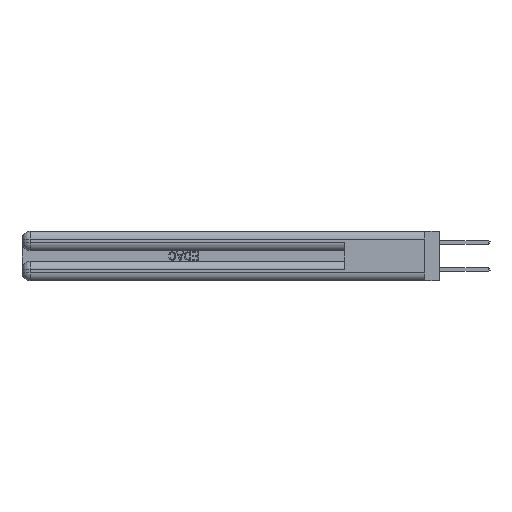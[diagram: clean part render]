
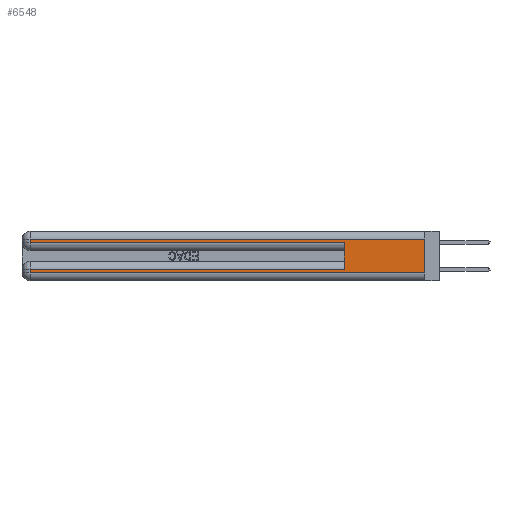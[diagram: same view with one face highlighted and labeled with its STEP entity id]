
A CAD part, left-side view. The second image highlights one B-rep face of the part: STEP entity #6548.
In plain terms, the highlighted planar face has unit normal (-1, 0, 0).
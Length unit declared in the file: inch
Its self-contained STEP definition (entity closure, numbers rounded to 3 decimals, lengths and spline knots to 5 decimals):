
#258 = LINE ( 'NONE', #27085, #29530 ) ;
#1089 = VERTEX_POINT ( 'NONE', #24024 ) ;
#1900 = VERTEX_POINT ( 'NONE', #43409 ) ;
#3963 = VECTOR ( 'NONE', #14091, 39.37008 ) ;
#4613 = CARTESIAN_POINT ( 'NONE',  ( 0., 0., 0.285 ) ) ;
#5064 = DIRECTION ( 'NONE',  ( 0., -1., 0. ) ) ;
#5409 = VERTEX_POINT ( 'NONE', #17122 ) ;
#6548 = ADVANCED_FACE ( 'NONE', ( #34229 ), #28766, .F. ) ;
#7283 = ORIENTED_EDGE ( 'NONE', *, *, #45114, .T. ) ;
#7579 = EDGE_CURVE ( 'NONE', #17850, #36302, #11174, .T. ) ;
#8300 = DIRECTION ( 'NONE',  ( 0., -1., 0. ) ) ;
#8536 = EDGE_LOOP ( 'NONE', ( #27753, #34011, #43330, #7283, #33862, #44814, #28402, #41227 ) ) ;
#9392 = DIRECTION ( 'NONE',  ( 0., 1., 0. ) ) ;
#9418 = EDGE_CURVE ( 'NONE', #31001, #5409, #35344, .T. ) ;
#10345 = CARTESIAN_POINT ( 'NONE',  ( 0., 0., 0.31 ) ) ;
#10462 = DIRECTION ( 'NONE',  ( 0., 0., -1. ) ) ;
#11174 = LINE ( 'NONE', #46698, #30667 ) ;
#11212 = EDGE_CURVE ( 'NONE', #1900, #1089, #258, .T. ) ;
#12594 = CARTESIAN_POINT ( 'NONE',  ( 0., 0.6, 0.145 ) ) ;
#12861 = VECTOR ( 'NONE', #8300, 39.37008 ) ;
#13589 = VERTEX_POINT ( 'NONE', #28543 ) ;
#14091 = DIRECTION ( 'NONE',  ( 0., 1., 0. ) ) ;
#15012 = CARTESIAN_POINT ( 'NONE',  ( 0., 2.94, 0.285 ) ) ;
#15238 = VERTEX_POINT ( 'NONE', #45117 ) ;
#15394 = LINE ( 'NONE', #41301, #33690 ) ;
#17037 = EDGE_CURVE ( 'NONE', #15238, #1089, #15394, .T. ) ;
#17122 = CARTESIAN_POINT ( 'NONE',  ( 0., 2.94, 0.085 ) ) ;
#17517 = DIRECTION ( 'NONE',  ( 0., 0., -1. ) ) ;
#17767 = CARTESIAN_POINT ( 'NONE',  ( 0., 0., 0.37 ) ) ;
#17850 = VERTEX_POINT ( 'NONE', #24314 ) ;
#20043 = DIRECTION ( 'NONE',  ( 0., 0., 1. ) ) ;
#20047 = EDGE_CURVE ( 'NONE', #5409, #1900, #39199, .T. ) ;
#20889 = DIRECTION ( 'NONE',  ( 0., 0., -1. ) ) ;
#22675 = LINE ( 'NONE', #4613, #12861 ) ;
#24024 = CARTESIAN_POINT ( 'NONE',  ( 0., 0., 0.06 ) ) ;
#24314 = CARTESIAN_POINT ( 'NONE',  ( 0., 2.94, 0.31 ) ) ;
#25640 = VECTOR ( 'NONE', #9392, 39.37008 ) ;
#26777 = DIRECTION ( 'NONE',  ( 0., 0., -1. ) ) ;
#27085 = CARTESIAN_POINT ( 'NONE',  ( 0., 0., 0.06 ) ) ;
#27753 = ORIENTED_EDGE ( 'NONE', *, *, #17037, .F. ) ;
#28315 = VECTOR ( 'NONE', #20889, 39.37008 ) ;
#28402 = ORIENTED_EDGE ( 'NONE', *, *, #20047, .T. ) ;
#28543 = CARTESIAN_POINT ( 'NONE',  ( 0., 0.6, 0.285 ) ) ;
#28766 = PLANE ( 'NONE',  #33378 ) ;
#29530 = VECTOR ( 'NONE', #5064, 39.37008 ) ;
#29612 = CARTESIAN_POINT ( 'NONE',  ( 0., 0.6, 0.085 ) ) ;
#30556 = VECTOR ( 'NONE', #20043, 39.37008 ) ;
#30667 = VECTOR ( 'NONE', #17517, 39.37008 ) ;
#31001 = VERTEX_POINT ( 'NONE', #29612 ) ;
#32430 = DIRECTION ( 'NONE',  ( 1., 0., 0. ) ) ;
#33378 = AXIS2_PLACEMENT_3D ( 'NONE', #17767, #32430, #10462 ) ;
#33690 = VECTOR ( 'NONE', #26777, 39.37008 ) ;
#33862 = ORIENTED_EDGE ( 'NONE', *, *, #45800, .F. ) ;
#34011 = ORIENTED_EDGE ( 'NONE', *, *, #39754, .T. ) ;
#34229 = FACE_OUTER_BOUND ( 'NONE', #8536, .T. ) ;
#35344 = LINE ( 'NONE', #38728, #25640 ) ;
#36302 = VERTEX_POINT ( 'NONE', #15012 ) ;
#38728 = CARTESIAN_POINT ( 'NONE',  ( 0., 0., 0.085 ) ) ;
#39199 = LINE ( 'NONE', #42891, #28315 ) ;
#39754 = EDGE_CURVE ( 'NONE', #15238, #17850, #42967, .T. ) ;
#40299 = LINE ( 'NONE', #12594, #30556 ) ;
#41227 = ORIENTED_EDGE ( 'NONE', *, *, #11212, .T. ) ;
#41301 = CARTESIAN_POINT ( 'NONE',  ( 0., 0., 0.37 ) ) ;
#42891 = CARTESIAN_POINT ( 'NONE',  ( 0., 2.94, 0.37 ) ) ;
#42967 = LINE ( 'NONE', #10345, #3963 ) ;
#43330 = ORIENTED_EDGE ( 'NONE', *, *, #7579, .T. ) ;
#43409 = CARTESIAN_POINT ( 'NONE',  ( 0., 2.94, 0.06 ) ) ;
#44814 = ORIENTED_EDGE ( 'NONE', *, *, #9418, .T. ) ;
#45114 = EDGE_CURVE ( 'NONE', #36302, #13589, #22675, .T. ) ;
#45117 = CARTESIAN_POINT ( 'NONE',  ( 0., 0., 0.31 ) ) ;
#45800 = EDGE_CURVE ( 'NONE', #31001, #13589, #40299, .T. ) ;
#46698 = CARTESIAN_POINT ( 'NONE',  ( 0., 2.94, 0.37 ) ) ;
